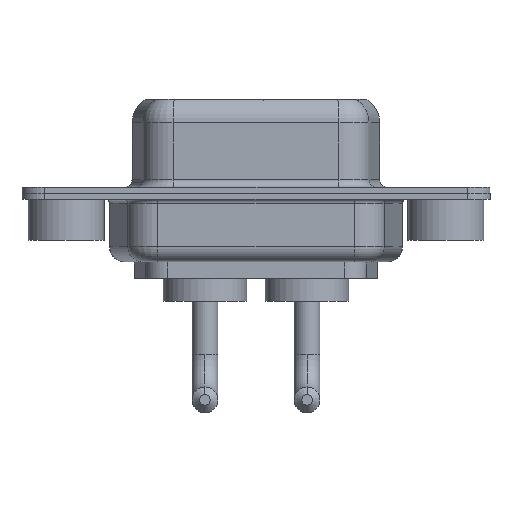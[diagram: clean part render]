
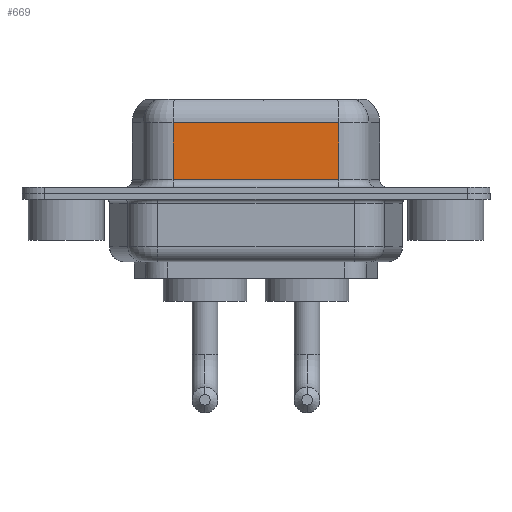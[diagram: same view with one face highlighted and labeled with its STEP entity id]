
A CAD part, front view. The second image highlights one B-rep face of the part: STEP entity #669.
In plain terms, the highlighted planar face has unit normal (0, -1, 0).
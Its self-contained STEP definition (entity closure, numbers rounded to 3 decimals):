
#190 = ORIENTED_EDGE ( 'NONE', *, *, #8114, .T. ) ;
#669 = ADVANCED_FACE ( 'NONE', ( #11237 ), #6327, .F. ) ;
#1040 = CARTESIAN_POINT ( 'NONE',  ( 7.038, -3.95, 6.4 ) ) ;
#1384 = EDGE_CURVE ( 'NONE', #10524, #12258, #7220, .T. ) ;
#1583 = EDGE_LOOP ( 'NONE', ( #7174, #190, #9328, #5361 ) ) ;
#1964 = LINE ( 'NONE', #6059, #3815 ) ;
#2209 = DIRECTION ( 'NONE',  ( 1., 0., 0. ) ) ;
#2230 = CARTESIAN_POINT ( 'NONE',  ( 17.962, -3.95, 6.4 ) ) ;
#2709 = CARTESIAN_POINT ( 'NONE',  ( 17.962, -3.95, 0.9 ) ) ;
#2818 = DIRECTION ( 'NONE',  ( -1., 0., 0. ) ) ;
#3196 = VERTEX_POINT ( 'NONE', #2709 ) ;
#3815 = VECTOR ( 'NONE', #10157, 1000. ) ;
#4080 = VECTOR ( 'NONE', #9997, 1000. ) ;
#4233 = DIRECTION ( 'NONE',  ( 0., 1., 0. ) ) ;
#5031 = CARTESIAN_POINT ( 'NONE',  ( 17.962, -3.95, 0.9 ) ) ;
#5361 = ORIENTED_EDGE ( 'NONE', *, *, #11039, .T. ) ;
#5736 = CARTESIAN_POINT ( 'NONE',  ( 17.962, -3.95, 4.65 ) ) ;
#6059 = CARTESIAN_POINT ( 'NONE',  ( 17.962, -3.95, 6.4 ) ) ;
#6178 = LINE ( 'NONE', #5031, #11522 ) ;
#6327 = PLANE ( 'NONE',  #9664 ) ;
#7174 = ORIENTED_EDGE ( 'NONE', *, *, #7748, .F. ) ;
#7220 = LINE ( 'NONE', #1040, #4080 ) ;
#7748 = EDGE_CURVE ( 'NONE', #9420, #3196, #1964, .T. ) ;
#8114 = EDGE_CURVE ( 'NONE', #9420, #10524, #13163, .T. ) ;
#8341 = CARTESIAN_POINT ( 'NONE',  ( 7.038, -3.95, 4.65 ) ) ;
#9328 = ORIENTED_EDGE ( 'NONE', *, *, #1384, .T. ) ;
#9420 = VERTEX_POINT ( 'NONE', #5736 ) ;
#9664 = AXIS2_PLACEMENT_3D ( 'NONE', #2230, #4233, #10226 ) ;
#9997 = DIRECTION ( 'NONE',  ( 0., 0., -1. ) ) ;
#10157 = DIRECTION ( 'NONE',  ( 0., 0., -1. ) ) ;
#10226 = DIRECTION ( 'NONE',  ( -1., 0., 0. ) ) ;
#10524 = VERTEX_POINT ( 'NONE', #8341 ) ;
#10782 = CARTESIAN_POINT ( 'NONE',  ( 7.038, -3.95, 0.9 ) ) ;
#10946 = CARTESIAN_POINT ( 'NONE',  ( 17.962, -3.95, 4.65 ) ) ;
#11039 = EDGE_CURVE ( 'NONE', #12258, #3196, #6178, .T. ) ;
#11237 = FACE_OUTER_BOUND ( 'NONE', #1583, .T. ) ;
#11522 = VECTOR ( 'NONE', #2209, 1000. ) ;
#12258 = VERTEX_POINT ( 'NONE', #10782 ) ;
#13163 = LINE ( 'NONE', #10946, #13277 ) ;
#13277 = VECTOR ( 'NONE', #2818, 1000. ) ;
